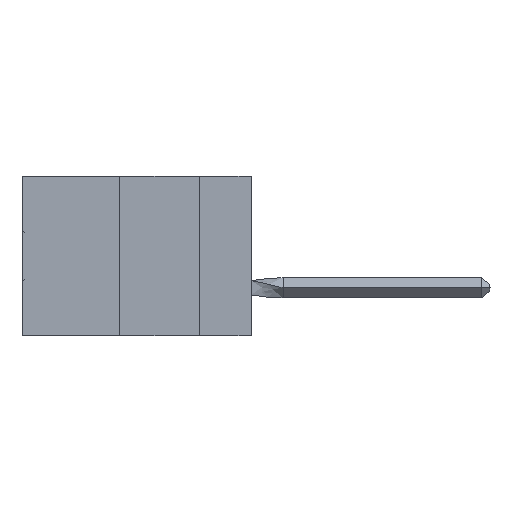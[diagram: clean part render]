
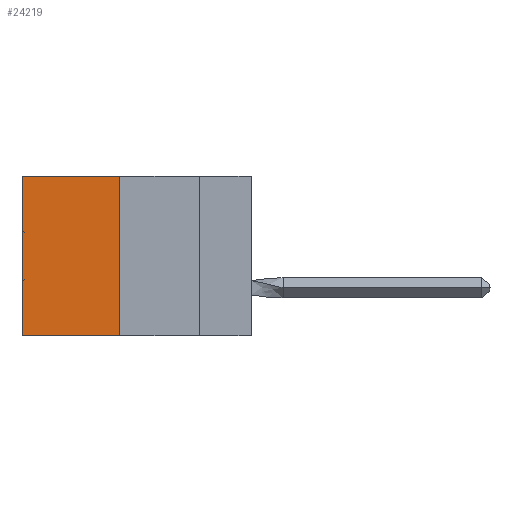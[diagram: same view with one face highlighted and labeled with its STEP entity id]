
A CAD part, left-side view. The second image highlights one B-rep face of the part: STEP entity #24219.
In plain terms, the highlighted planar face has unit normal (-1, 0, 0).
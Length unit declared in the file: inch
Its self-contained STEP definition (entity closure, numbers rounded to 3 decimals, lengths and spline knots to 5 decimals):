
#947 = VECTOR ( 'NONE', #12743, 39.37008 ) ;
#3115 = EDGE_CURVE ( 'NONE', #17594, #25712, #15484, .T. ) ;
#3857 = DIRECTION ( 'NONE',  ( 0., 1., 0. ) ) ;
#4154 = EDGE_CURVE ( 'NONE', #20830, #17594, #34432, .T. ) ;
#6885 = ORIENTED_EDGE ( 'NONE', *, *, #3115, .F. ) ;
#8790 = CARTESIAN_POINT ( 'NONE',  ( 0.305, 0.72, -0.5 ) ) ;
#8922 = VECTOR ( 'NONE', #30251, 39.37008 ) ;
#11692 = AXIS2_PLACEMENT_3D ( 'NONE', #45492, #19895, #24508 ) ;
#12373 = FACE_OUTER_BOUND ( 'NONE', #47129, .T. ) ;
#12743 = DIRECTION ( 'NONE',  ( 0., 0., -1. ) ) ;
#12847 = CARTESIAN_POINT ( 'NONE',  ( 0.305, 0.72, -0.5 ) ) ;
#13941 = ORIENTED_EDGE ( 'NONE', *, *, #4154, .F. ) ;
#15484 = LINE ( 'NONE', #29597, #52331 ) ;
#17594 = VERTEX_POINT ( 'NONE', #43325 ) ;
#19895 = DIRECTION ( 'NONE',  ( 1., 0., 0. ) ) ;
#20027 = EDGE_CURVE ( 'NONE', #20830, #22226, #48560, .T. ) ;
#20830 = VERTEX_POINT ( 'NONE', #31442 ) ;
#22226 = VERTEX_POINT ( 'NONE', #24805 ) ;
#23540 = VECTOR ( 'NONE', #27129, 39.37008 ) ;
#23807 = ORIENTED_EDGE ( 'NONE', *, *, #31334, .T. ) ;
#24219 = ADVANCED_FACE ( 'NONE', ( #12373 ), #40726, .F. ) ;
#24508 = DIRECTION ( 'NONE',  ( 0., 0., -1. ) ) ;
#24805 = CARTESIAN_POINT ( 'NONE',  ( 0.305, 0.72, 0. ) ) ;
#25712 = VERTEX_POINT ( 'NONE', #12847 ) ;
#27129 = DIRECTION ( 'NONE',  ( 0., 1., 0. ) ) ;
#27245 = LINE ( 'NONE', #8790, #8922 ) ;
#29597 = CARTESIAN_POINT ( 'NONE',  ( 0.305, 0.413, -0.5 ) ) ;
#30251 = DIRECTION ( 'NONE',  ( 0., 0., -1. ) ) ;
#31334 = EDGE_CURVE ( 'NONE', #22226, #25712, #27245, .T. ) ;
#31442 = CARTESIAN_POINT ( 'NONE',  ( 0.305, 0.413, 0. ) ) ;
#34432 = LINE ( 'NONE', #50397, #947 ) ;
#35205 = CARTESIAN_POINT ( 'NONE',  ( 0.305, 0.413, 0. ) ) ;
#40726 = PLANE ( 'NONE',  #11692 ) ;
#43325 = CARTESIAN_POINT ( 'NONE',  ( 0.305, 0.413, -0.5 ) ) ;
#45492 = CARTESIAN_POINT ( 'NONE',  ( 0.305, 0.413, -0.5 ) ) ;
#47129 = EDGE_LOOP ( 'NONE', ( #23807, #6885, #13941, #49450 ) ) ;
#48560 = LINE ( 'NONE', #35205, #23540 ) ;
#49450 = ORIENTED_EDGE ( 'NONE', *, *, #20027, .T. ) ;
#50397 = CARTESIAN_POINT ( 'NONE',  ( 0.305, 0.413, -0.5 ) ) ;
#52331 = VECTOR ( 'NONE', #3857, 39.37008 ) ;
